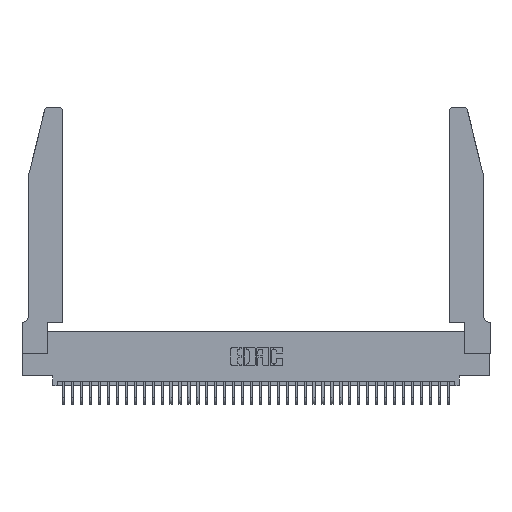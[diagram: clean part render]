
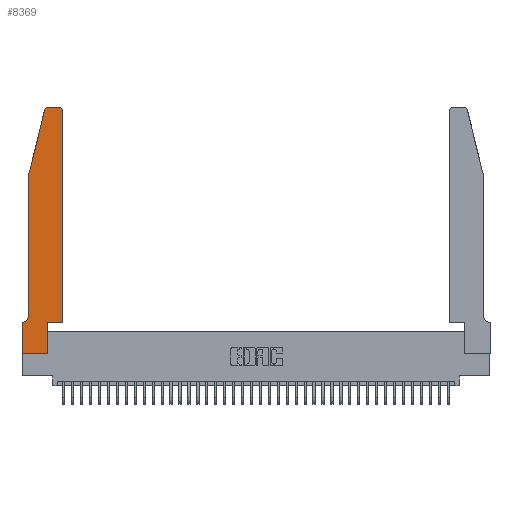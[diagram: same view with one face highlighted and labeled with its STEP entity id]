
A CAD part, top view. The second image highlights one B-rep face of the part: STEP entity #8369.
In plain terms, the highlighted planar face has unit normal (0, 0, 1).
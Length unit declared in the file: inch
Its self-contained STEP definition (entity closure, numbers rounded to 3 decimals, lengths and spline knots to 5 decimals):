
#51 = DIRECTION ( 'NONE',  ( -1., 0., 0. ) ) ;
#136 = VERTEX_POINT ( 'NONE', #22643 ) ;
#805 = VERTEX_POINT ( 'NONE', #27684 ) ;
#1392 = CARTESIAN_POINT ( 'NONE',  ( 0.284, 2.72, 0.37 ) ) ;
#1653 = VERTEX_POINT ( 'NONE', #6099 ) ;
#1822 = VECTOR ( 'NONE', #14906, 39.37008 ) ;
#2491 = ORIENTED_EDGE ( 'NONE', *, *, #27850, .T. ) ;
#3409 = LINE ( 'NONE', #3670, #38453 ) ;
#3531 = ORIENTED_EDGE ( 'NONE', *, *, #28019, .T. ) ;
#3571 = VECTOR ( 'NONE', #28517, 39.37008 ) ;
#3670 = CARTESIAN_POINT ( 'NONE',  ( 0.4505, 0.35, 0.37 ) ) ;
#5266 = CARTESIAN_POINT ( 'NONE',  ( 0.2605, 2.75, 0.37 ) ) ;
#5780 = CARTESIAN_POINT ( 'NONE',  ( 0.2865, 0.35, 0.37 ) ) ;
#6068 = VERTEX_POINT ( 'NONE', #18236 ) ;
#6099 = CARTESIAN_POINT ( 'NONE',  ( 0., 0.35, 0.37 ) ) ;
#7443 = CARTESIAN_POINT ( 'NONE',  ( 0.4505, 0.35, 0.37 ) ) ;
#7819 = EDGE_CURVE ( 'NONE', #13051, #31599, #9808, .T. ) ;
#7824 = EDGE_CURVE ( 'NONE', #15703, #13051, #3409, .T. ) ;
#8110 = LINE ( 'NONE', #5266, #36735 ) ;
#8369 = ADVANCED_FACE ( 'NONE', ( #37433 ), #36837, .T. ) ;
#8550 = EDGE_CURVE ( 'NONE', #8818, #1653, #27529, .T. ) ;
#8818 = VERTEX_POINT ( 'NONE', #33869 ) ;
#9808 = LINE ( 'NONE', #25774, #23648 ) ;
#10029 = AXIS2_PLACEMENT_3D ( 'NONE', #34115, #28165, #15169 ) ;
#10037 = CARTESIAN_POINT ( 'NONE',  ( 0.2865, 0., 0.37 ) ) ;
#10587 = DIRECTION ( 'NONE',  ( 0., -1., 0. ) ) ;
#11343 = CARTESIAN_POINT ( 'NONE',  ( 0.4505, 2.72, 0.37 ) ) ;
#11691 = DIRECTION ( 'NONE',  ( 0., 1., 0. ) ) ;
#12226 = CARTESIAN_POINT ( 'NONE',  ( 0.0755, 0.42, 0.37 ) ) ;
#12532 = CIRCLE ( 'NONE', #39205, 0.03 ) ;
#12760 = DIRECTION ( 'NONE',  ( 0., -1., 0. ) ) ;
#13049 = VERTEX_POINT ( 'NONE', #28975 ) ;
#13051 = VERTEX_POINT ( 'NONE', #7443 ) ;
#13483 = CARTESIAN_POINT ( 'NONE',  ( 0.0055, 0.42, 0.37 ) ) ;
#14865 = DIRECTION ( 'NONE',  ( 0., 0., 1. ) ) ;
#14906 = DIRECTION ( 'NONE',  ( -1., 0., 0. ) ) ;
#15010 = CARTESIAN_POINT ( 'NONE',  ( 0., 0.35, 0.37 ) ) ;
#15134 = ORIENTED_EDGE ( 'NONE', *, *, #30353, .T. ) ;
#15169 = DIRECTION ( 'NONE',  ( 1., 0., 0. ) ) ;
#15337 = EDGE_CURVE ( 'NONE', #16344, #15703, #39870, .T. ) ;
#15703 = VERTEX_POINT ( 'NONE', #40119 ) ;
#15727 = VECTOR ( 'NONE', #10587, 39.37008 ) ;
#16344 = VERTEX_POINT ( 'NONE', #10037 ) ;
#16615 = ORIENTED_EDGE ( 'NONE', *, *, #25330, .T. ) ;
#17292 = AXIS2_PLACEMENT_3D ( 'NONE', #15010, #14865, #21372 ) ;
#17692 = LINE ( 'NONE', #26759, #15727 ) ;
#18017 = EDGE_CURVE ( 'NONE', #28729, #31101, #29756, .T. ) ;
#18236 = CARTESIAN_POINT ( 'NONE',  ( 0.4205, 2.75, 0.37 ) ) ;
#19015 = CARTESIAN_POINT ( 'NONE',  ( 0., 0., 0.37 ) ) ;
#19535 = DIRECTION ( 'NONE',  ( 1., 0., 0. ) ) ;
#20160 = VECTOR ( 'NONE', #11691, 39.37008 ) ;
#20868 = CARTESIAN_POINT ( 'NONE',  ( 0.0755, 0.35, 0.37 ) ) ;
#20885 = ORIENTED_EDGE ( 'NONE', *, *, #8550, .T. ) ;
#21372 = DIRECTION ( 'NONE',  ( 1., 0., 0. ) ) ;
#22024 = ORIENTED_EDGE ( 'NONE', *, *, #23060, .T. ) ;
#22243 = ORIENTED_EDGE ( 'NONE', *, *, #15337, .T. ) ;
#22389 = ORIENTED_EDGE ( 'NONE', *, *, #7819, .T. ) ;
#22643 = CARTESIAN_POINT ( 'NONE',  ( 0.284, 2.75, 0.37 ) ) ;
#22714 = DIRECTION ( 'NONE',  ( 0., 1., 0. ) ) ;
#22752 = DIRECTION ( 'NONE',  ( 0., 0., -1. ) ) ;
#23060 = EDGE_CURVE ( 'NONE', #6068, #136, #8110, .T. ) ;
#23192 = EDGE_CURVE ( 'NONE', #136, #805, #12532, .T. ) ;
#23591 = DIRECTION ( 'NONE',  ( 0., 0., 1. ) ) ;
#23648 = VECTOR ( 'NONE', #22714, 39.37008 ) ;
#24710 = ORIENTED_EDGE ( 'NONE', *, *, #23192, .T. ) ;
#25330 = EDGE_CURVE ( 'NONE', #13049, #16344, #28751, .T. ) ;
#25404 = VECTOR ( 'NONE', #39577, 39.37008 ) ;
#25774 = CARTESIAN_POINT ( 'NONE',  ( 0.4505, 0.35, 0.37 ) ) ;
#26759 = CARTESIAN_POINT ( 'NONE',  ( 0., 0., 0.37 ) ) ;
#26854 = LINE ( 'NONE', #26927, #25404 ) ;
#26927 = CARTESIAN_POINT ( 'NONE',  ( 0.0755, 2., 0.37 ) ) ;
#27529 = LINE ( 'NONE', #20868, #1822 ) ;
#27568 = CIRCLE ( 'NONE', #39564, 0.07 ) ;
#27684 = CARTESIAN_POINT ( 'NONE',  ( 0.25487, 2.72718, 0.37 ) ) ;
#27850 = EDGE_CURVE ( 'NONE', #31101, #8818, #27568, .T. ) ;
#28019 = EDGE_CURVE ( 'NONE', #1653, #13049, #17692, .T. ) ;
#28035 = EDGE_LOOP ( 'NONE', ( #22024, #24710, #31238, #40613, #2491, #20885, #3531, #16615, #22243, #31860, #22389, #15134 ) ) ;
#28165 = DIRECTION ( 'NONE',  ( 0., 0., 1. ) ) ;
#28517 = DIRECTION ( 'NONE',  ( 1., 0., 0. ) ) ;
#28729 = VERTEX_POINT ( 'NONE', #30267 ) ;
#28751 = LINE ( 'NONE', #19015, #3571 ) ;
#28975 = CARTESIAN_POINT ( 'NONE',  ( 0., 0., 0.37 ) ) ;
#29756 = LINE ( 'NONE', #37783, #35207 ) ;
#30267 = CARTESIAN_POINT ( 'NONE',  ( 0.0755, 2., 0.37 ) ) ;
#30353 = EDGE_CURVE ( 'NONE', #31599, #6068, #30825, .T. ) ;
#30825 = CIRCLE ( 'NONE', #10029, 0.03 ) ;
#31101 = VERTEX_POINT ( 'NONE', #12226 ) ;
#31238 = ORIENTED_EDGE ( 'NONE', *, *, #33960, .T. ) ;
#31599 = VERTEX_POINT ( 'NONE', #11343 ) ;
#31860 = ORIENTED_EDGE ( 'NONE', *, *, #7824, .T. ) ;
#31995 = DIRECTION ( 'NONE',  ( -1., 0., 0. ) ) ;
#33244 = DIRECTION ( 'NONE',  ( 1., 0., 0. ) ) ;
#33869 = CARTESIAN_POINT ( 'NONE',  ( 0.0055, 0.35, 0.37 ) ) ;
#33960 = EDGE_CURVE ( 'NONE', #805, #28729, #26854, .T. ) ;
#34115 = CARTESIAN_POINT ( 'NONE',  ( 0.4205, 2.72, 0.37 ) ) ;
#35207 = VECTOR ( 'NONE', #12760, 39.37008 ) ;
#36735 = VECTOR ( 'NONE', #51, 39.37008 ) ;
#36837 = PLANE ( 'NONE',  #17292 ) ;
#37433 = FACE_OUTER_BOUND ( 'NONE', #28035, .T. ) ;
#37783 = CARTESIAN_POINT ( 'NONE',  ( 0.0755, 2., 0.37 ) ) ;
#38453 = VECTOR ( 'NONE', #19535, 39.37008 ) ;
#39205 = AXIS2_PLACEMENT_3D ( 'NONE', #1392, #23591, #33244 ) ;
#39564 = AXIS2_PLACEMENT_3D ( 'NONE', #13483, #22752, #31995 ) ;
#39577 = DIRECTION ( 'NONE',  ( -0.239, -0.971, 0. ) ) ;
#39870 = LINE ( 'NONE', #5780, #20160 ) ;
#40119 = CARTESIAN_POINT ( 'NONE',  ( 0.2865, 0.35, 0.37 ) ) ;
#40613 = ORIENTED_EDGE ( 'NONE', *, *, #18017, .T. ) ;
